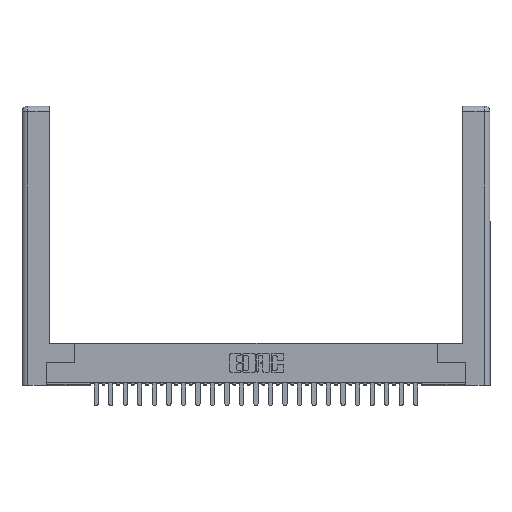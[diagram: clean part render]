
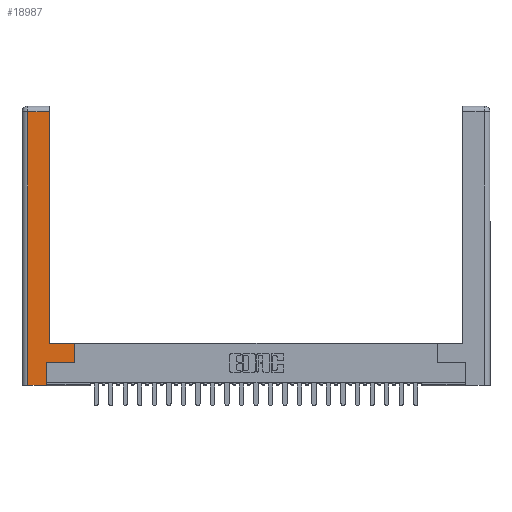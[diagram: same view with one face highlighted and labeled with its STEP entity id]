
A CAD part, top view. The second image highlights one B-rep face of the part: STEP entity #18987.
In plain terms, the highlighted planar face has unit normal (0, 0, 1).
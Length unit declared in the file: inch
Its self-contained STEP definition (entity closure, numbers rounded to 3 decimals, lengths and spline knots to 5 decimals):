
#273 = VECTOR ( 'NONE', #27116, 39.37008 ) ;
#491 = CARTESIAN_POINT ( 'NONE',  ( 0.265, 0., 0. ) ) ;
#995 = VERTEX_POINT ( 'NONE', #24292 ) ;
#1074 = ORIENTED_EDGE ( 'NONE', *, *, #25966, .T. ) ;
#1428 = CARTESIAN_POINT ( 'NONE',  ( 0.295, 2.94, 0. ) ) ;
#1814 = ORIENTED_EDGE ( 'NONE', *, *, #27965, .T. ) ;
#1906 = LINE ( 'NONE', #20949, #5505 ) ;
#4074 = CARTESIAN_POINT ( 'NONE',  ( 0.0615, 2.94, 0. ) ) ;
#4353 = CARTESIAN_POINT ( 'NONE',  ( 0.565, 0.245, 0. ) ) ;
#5505 = VECTOR ( 'NONE', #27626, 39.37008 ) ;
#5570 = ORIENTED_EDGE ( 'NONE', *, *, #10211, .T. ) ;
#5986 = ORIENTED_EDGE ( 'NONE', *, *, #28849, .T. ) ;
#6022 = VECTOR ( 'NONE', #13486, 39.37008 ) ;
#6563 = DIRECTION ( 'NONE',  ( -1., 0., 0. ) ) ;
#7127 = LINE ( 'NONE', #8103, #11421 ) ;
#7156 = VECTOR ( 'NONE', #18194, 39.37008 ) ;
#7285 = VERTEX_POINT ( 'NONE', #4074 ) ;
#7953 = EDGE_CURVE ( 'NONE', #29177, #995, #22179, .T. ) ;
#8103 = CARTESIAN_POINT ( 'NONE',  ( 0.295, 0.45, 0. ) ) ;
#8435 = DIRECTION ( 'NONE',  ( 1., 0., 0. ) ) ;
#8851 = CARTESIAN_POINT ( 'NONE',  ( 0.0615, 2.94, 0. ) ) ;
#9693 = ORIENTED_EDGE ( 'NONE', *, *, #18191, .T. ) ;
#9983 = VECTOR ( 'NONE', #15178, 39.37008 ) ;
#10211 = EDGE_CURVE ( 'NONE', #19011, #24684, #29312, .T. ) ;
#10393 = VERTEX_POINT ( 'NONE', #20952 ) ;
#10730 = LINE ( 'NONE', #8851, #7156 ) ;
#11167 = CARTESIAN_POINT ( 'NONE',  ( 0.295, 0.45, 0. ) ) ;
#11348 = EDGE_CURVE ( 'NONE', #23741, #19011, #7127, .T. ) ;
#11421 = VECTOR ( 'NONE', #21911, 39.37008 ) ;
#12206 = EDGE_LOOP ( 'NONE', ( #5570, #1814, #5986, #29033, #24507, #9693, #1074, #19924 ) ) ;
#12811 = LINE ( 'NONE', #18053, #6022 ) ;
#12878 = CARTESIAN_POINT ( 'NONE',  ( 0.265, 0.245, 0. ) ) ;
#13486 = DIRECTION ( 'NONE',  ( 0., -1., 0. ) ) ;
#14571 = EDGE_CURVE ( 'NONE', #24477, #29177, #23430, .T. ) ;
#14854 = FACE_OUTER_BOUND ( 'NONE', #12206, .T. ) ;
#15178 = DIRECTION ( 'NONE',  ( 0., 1., 0. ) ) ;
#15192 = AXIS2_PLACEMENT_3D ( 'NONE', #15363, #29275, #6563 ) ;
#15363 = CARTESIAN_POINT ( 'NONE',  ( 0., 0., 0. ) ) ;
#17559 = CARTESIAN_POINT ( 'NONE',  ( 0.565, 0.45, 0. ) ) ;
#18053 = CARTESIAN_POINT ( 'NONE',  ( 0.0615, 0., 0. ) ) ;
#18191 = EDGE_CURVE ( 'NONE', #995, #10393, #21727, .T. ) ;
#18194 = DIRECTION ( 'NONE',  ( -1., 0., 0. ) ) ;
#18987 = ADVANCED_FACE ( 'NONE', ( #14854 ), #22501, .F. ) ;
#19011 = VERTEX_POINT ( 'NONE', #11167 ) ;
#19924 = ORIENTED_EDGE ( 'NONE', *, *, #11348, .T. ) ;
#20949 = CARTESIAN_POINT ( 'NONE',  ( 0.565, 0.45, 0. ) ) ;
#20952 = CARTESIAN_POINT ( 'NONE',  ( 0.565, 0.245, 0. ) ) ;
#20988 = CARTESIAN_POINT ( 'NONE',  ( 0.295, 3., 0. ) ) ;
#21727 = LINE ( 'NONE', #4353, #273 ) ;
#21911 = DIRECTION ( 'NONE',  ( -1., 0., 0. ) ) ;
#22179 = LINE ( 'NONE', #12878, #9983 ) ;
#22501 = PLANE ( 'NONE',  #15192 ) ;
#23068 = VECTOR ( 'NONE', #8435, 39.37008 ) ;
#23430 = LINE ( 'NONE', #29374, #23068 ) ;
#23741 = VERTEX_POINT ( 'NONE', #17559 ) ;
#24292 = CARTESIAN_POINT ( 'NONE',  ( 0.265, 0.245, 0. ) ) ;
#24477 = VERTEX_POINT ( 'NONE', #27256 ) ;
#24507 = ORIENTED_EDGE ( 'NONE', *, *, #7953, .T. ) ;
#24684 = VERTEX_POINT ( 'NONE', #1428 ) ;
#25966 = EDGE_CURVE ( 'NONE', #10393, #23741, #1906, .T. ) ;
#26305 = DIRECTION ( 'NONE',  ( 0., 1., 0. ) ) ;
#27116 = DIRECTION ( 'NONE',  ( 1., 0., 0. ) ) ;
#27256 = CARTESIAN_POINT ( 'NONE',  ( 0.0615, 0., 0. ) ) ;
#27626 = DIRECTION ( 'NONE',  ( 0., 1., 0. ) ) ;
#27965 = EDGE_CURVE ( 'NONE', #24684, #7285, #10730, .T. ) ;
#28849 = EDGE_CURVE ( 'NONE', #7285, #24477, #12811, .T. ) ;
#28963 = VECTOR ( 'NONE', #26305, 39.37008 ) ;
#29033 = ORIENTED_EDGE ( 'NONE', *, *, #14571, .T. ) ;
#29177 = VERTEX_POINT ( 'NONE', #491 ) ;
#29275 = DIRECTION ( 'NONE',  ( 0., 0., -1. ) ) ;
#29312 = LINE ( 'NONE', #20988, #28963 ) ;
#29374 = CARTESIAN_POINT ( 'NONE',  ( 0.265, 0., 0. ) ) ;
